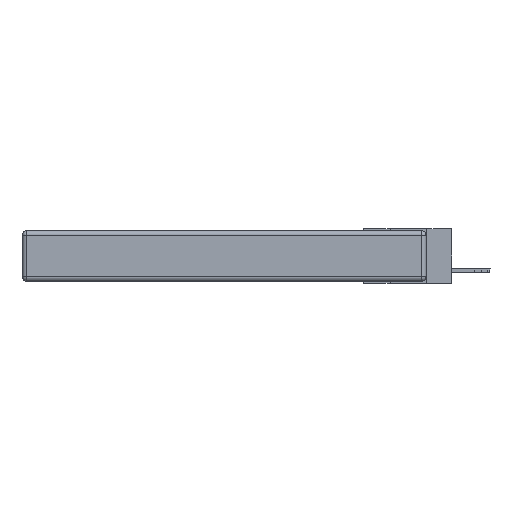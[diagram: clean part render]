
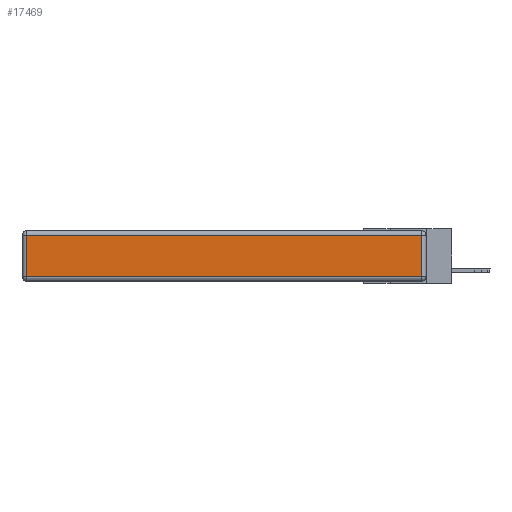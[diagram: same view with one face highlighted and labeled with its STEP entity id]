
A CAD part, left-side view. The second image highlights one B-rep face of the part: STEP entity #17469.
In plain terms, the highlighted planar face has unit normal (-1, 0, 0).
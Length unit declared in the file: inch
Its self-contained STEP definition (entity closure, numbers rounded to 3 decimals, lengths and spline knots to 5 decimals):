
#110 = EDGE_CURVE ( 'NONE', #8801, #9531, #12135, .T. ) ;
#341 = VERTEX_POINT ( 'NONE', #14727 ) ;
#911 = ORIENTED_EDGE ( 'NONE', *, *, #11702, .T. ) ;
#1305 = DIRECTION ( 'NONE',  ( 0., -1., 0. ) ) ;
#1397 = CARTESIAN_POINT ( 'NONE',  ( 0., 0.03, -0.03 ) ) ;
#1525 = ORIENTED_EDGE ( 'NONE', *, *, #12960, .T. ) ;
#2037 = FACE_OUTER_BOUND ( 'NONE', #3492, .T. ) ;
#2540 = CARTESIAN_POINT ( 'NONE',  ( 0., 2.72, -0.343 ) ) ;
#2764 = CARTESIAN_POINT ( 'NONE',  ( 0., 0., -0.313 ) ) ;
#3492 = EDGE_LOOP ( 'NONE', ( #911, #1525, #15057, #9739 ) ) ;
#4515 = LINE ( 'NONE', #18937, #8713 ) ;
#6110 = CARTESIAN_POINT ( 'NONE',  ( 0., 2.72, -0.313 ) ) ;
#7369 = CARTESIAN_POINT ( 'NONE',  ( 0., 0., -0.343 ) ) ;
#7566 = DIRECTION ( 'NONE',  ( -1., 0., 0. ) ) ;
#8629 = VECTOR ( 'NONE', #15677, 39.37008 ) ;
#8667 = LINE ( 'NONE', #2764, #11919 ) ;
#8713 = VECTOR ( 'NONE', #15600, 39.37008 ) ;
#8750 = VECTOR ( 'NONE', #10325, 39.37008 ) ;
#8801 = VERTEX_POINT ( 'NONE', #1397 ) ;
#9531 = VERTEX_POINT ( 'NONE', #15236 ) ;
#9739 = ORIENTED_EDGE ( 'NONE', *, *, #17279, .T. ) ;
#9903 = AXIS2_PLACEMENT_3D ( 'NONE', #7369, #7566, #15569 ) ;
#10325 = DIRECTION ( 'NONE',  ( 0., 0., -1. ) ) ;
#10810 = PLANE ( 'NONE',  #9903 ) ;
#11702 = EDGE_CURVE ( 'NONE', #11828, #341, #8667, .T. ) ;
#11754 = LINE ( 'NONE', #2540, #8750 ) ;
#11828 = VERTEX_POINT ( 'NONE', #6110 ) ;
#11919 = VECTOR ( 'NONE', #1305, 39.37008 ) ;
#12135 = LINE ( 'NONE', #20399, #8629 ) ;
#12960 = EDGE_CURVE ( 'NONE', #341, #8801, #4515, .T. ) ;
#14727 = CARTESIAN_POINT ( 'NONE',  ( 0., 0.03, -0.313 ) ) ;
#15057 = ORIENTED_EDGE ( 'NONE', *, *, #110, .T. ) ;
#15236 = CARTESIAN_POINT ( 'NONE',  ( 0., 2.72, -0.03 ) ) ;
#15569 = DIRECTION ( 'NONE',  ( 0., 0., 1. ) ) ;
#15600 = DIRECTION ( 'NONE',  ( 0., 0., 1. ) ) ;
#15677 = DIRECTION ( 'NONE',  ( 0., 1., 0. ) ) ;
#17279 = EDGE_CURVE ( 'NONE', #9531, #11828, #11754, .T. ) ;
#17469 = ADVANCED_FACE ( 'NONE', ( #2037 ), #10810, .T. ) ;
#18937 = CARTESIAN_POINT ( 'NONE',  ( 0., 0.03, -0.343 ) ) ;
#20399 = CARTESIAN_POINT ( 'NONE',  ( 0., 2.75, -0.03 ) ) ;
